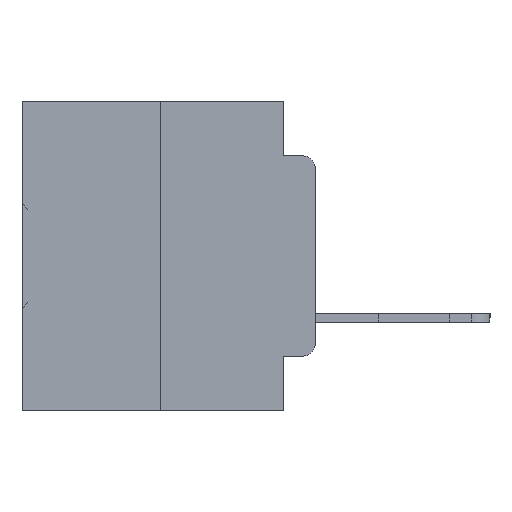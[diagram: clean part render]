
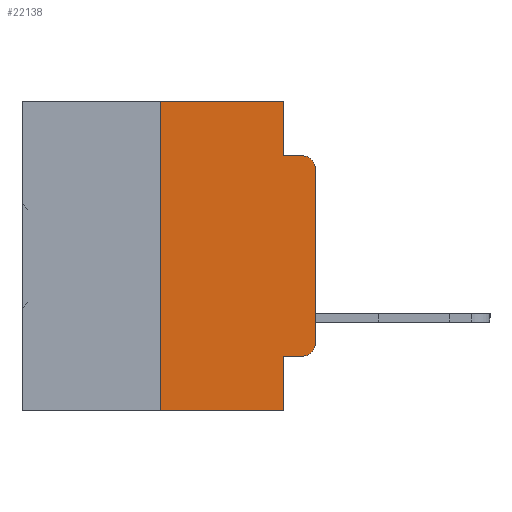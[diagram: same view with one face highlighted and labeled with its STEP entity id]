
A CAD part, left-side view. The second image highlights one B-rep face of the part: STEP entity #22138.
In plain terms, the highlighted planar face has unit normal (-1, 0, 0).
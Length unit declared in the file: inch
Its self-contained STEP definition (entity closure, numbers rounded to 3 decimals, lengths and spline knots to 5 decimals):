
#580 = EDGE_CURVE ( 'NONE', #10509, #17704, #13970, .T. ) ;
#830 = DIRECTION ( 'NONE',  ( -1., 0., 0. ) ) ;
#951 = CARTESIAN_POINT ( 'NONE',  ( 0., 0.02, -0.3915 ) ) ;
#1448 = DIRECTION ( 'NONE',  ( 0., -1., 0. ) ) ;
#2131 = CARTESIAN_POINT ( 'NONE',  ( 0., 0.02, -0.4115 ) ) ;
#2895 = ORIENTED_EDGE ( 'NONE', *, *, #25923, .T. ) ;
#2924 = CARTESIAN_POINT ( 'NONE',  ( 0., 0., -0.1085 ) ) ;
#3681 = DIRECTION ( 'NONE',  ( 0., 0., -1. ) ) ;
#4774 = EDGE_CURVE ( 'NONE', #26540, #25588, #20699, .T. ) ;
#5045 = ORIENTED_EDGE ( 'NONE', *, *, #9909, .F. ) ;
#5196 = AXIS2_PLACEMENT_3D ( 'NONE', #951, #20064, #3681 ) ;
#6168 = VERTEX_POINT ( 'NONE', #33645 ) ;
#6640 = CARTESIAN_POINT ( 'NONE',  ( 0., 0.051, -0.0885 ) ) ;
#6739 = DIRECTION ( 'NONE',  ( 0., 0., 1. ) ) ;
#6847 = LINE ( 'NONE', #20016, #34656 ) ;
#6907 = EDGE_CURVE ( 'NONE', #20873, #34679, #17604, .T. ) ;
#7668 = ORIENTED_EDGE ( 'NONE', *, *, #33949, .F. ) ;
#7806 = LINE ( 'NONE', #27912, #21412 ) ;
#9909 = EDGE_CURVE ( 'NONE', #29156, #6168, #7806, .T. ) ;
#10174 = CARTESIAN_POINT ( 'NONE',  ( 0., 0.051, -0.5 ) ) ;
#10509 = VERTEX_POINT ( 'NONE', #30494 ) ;
#11052 = CIRCLE ( 'NONE', #5196, 0.02 ) ;
#11458 = LINE ( 'NONE', #31200, #24952 ) ;
#12085 = CARTESIAN_POINT ( 'NONE',  ( 0., 0.473, 0. ) ) ;
#12644 = VECTOR ( 'NONE', #6739, 39.37008 ) ;
#13255 = EDGE_CURVE ( 'NONE', #6168, #20873, #11458, .T. ) ;
#13520 = CARTESIAN_POINT ( 'NONE',  ( 0., 0.25, 0. ) ) ;
#13668 = ORIENTED_EDGE ( 'NONE', *, *, #33540, .T. ) ;
#13970 = LINE ( 'NONE', #15401, #29102 ) ;
#14832 = DIRECTION ( 'NONE',  ( 1., 0., 0. ) ) ;
#15401 = CARTESIAN_POINT ( 'NONE',  ( 0., 0.473, -0.5 ) ) ;
#15784 = ORIENTED_EDGE ( 'NONE', *, *, #32378, .F. ) ;
#15901 = VECTOR ( 'NONE', #25900, 39.37008 ) ;
#16081 = ORIENTED_EDGE ( 'NONE', *, *, #17423, .T. ) ;
#16259 = DIRECTION ( 'NONE',  ( 0., 0., 1. ) ) ;
#17233 = CARTESIAN_POINT ( 'NONE',  ( 0., 0.02, -0.1085 ) ) ;
#17407 = VECTOR ( 'NONE', #16259, 39.37008 ) ;
#17423 = EDGE_CURVE ( 'NONE', #25588, #34679, #34330, .T. ) ;
#17454 = DIRECTION ( 'NONE',  ( 0., -1., 0. ) ) ;
#17604 = LINE ( 'NONE', #17841, #15901 ) ;
#17704 = VERTEX_POINT ( 'NONE', #10174 ) ;
#17841 = CARTESIAN_POINT ( 'NONE',  ( 0., 0.051, -0.0885 ) ) ;
#18745 = ORIENTED_EDGE ( 'NONE', *, *, #13255, .F. ) ;
#19548 = ORIENTED_EDGE ( 'NONE', *, *, #6907, .F. ) ;
#19931 = DIRECTION ( 'NONE',  ( 0., 0., -1. ) ) ;
#19958 = EDGE_LOOP ( 'NONE', ( #34484, #16081, #19548, #18745, #5045, #7668, #29201, #15784, #2895, #13668 ) ) ;
#20016 = CARTESIAN_POINT ( 'NONE',  ( 0., 0.051, 0. ) ) ;
#20064 = DIRECTION ( 'NONE',  ( -1., 0., 0. ) ) ;
#20319 = CARTESIAN_POINT ( 'NONE',  ( 0., 0., 0. ) ) ;
#20699 = LINE ( 'NONE', #20319, #12644 ) ;
#20700 = CARTESIAN_POINT ( 'NONE',  ( 0., 0.051, -0.4115 ) ) ;
#20873 = VERTEX_POINT ( 'NONE', #6640 ) ;
#21412 = VECTOR ( 'NONE', #33291, 39.37008 ) ;
#22138 = ADVANCED_FACE ( 'NONE', ( #26741 ), #30798, .F. ) ;
#22362 = VECTOR ( 'NONE', #17454, 39.37008 ) ;
#22830 = DIRECTION ( 'NONE',  ( 0., 0., -1. ) ) ;
#24526 = LINE ( 'NONE', #13520, #17407 ) ;
#24952 = VECTOR ( 'NONE', #33846, 39.37008 ) ;
#25272 = CARTESIAN_POINT ( 'NONE',  ( 0., 0.02, -0.0885 ) ) ;
#25588 = VERTEX_POINT ( 'NONE', #2924 ) ;
#25603 = AXIS2_PLACEMENT_3D ( 'NONE', #12085, #14832, #33545 ) ;
#25900 = DIRECTION ( 'NONE',  ( 0., -1., 0. ) ) ;
#25923 = EDGE_CURVE ( 'NONE', #32507, #30167, #29452, .T. ) ;
#26540 = VERTEX_POINT ( 'NONE', #33523 ) ;
#26741 = FACE_OUTER_BOUND ( 'NONE', #19958, .T. ) ;
#27790 = CARTESIAN_POINT ( 'NONE',  ( 0., 0.25, 0. ) ) ;
#27912 = CARTESIAN_POINT ( 'NONE',  ( 0., 0.473, 0. ) ) ;
#28824 = AXIS2_PLACEMENT_3D ( 'NONE', #17233, #830, #19931 ) ;
#29102 = VECTOR ( 'NONE', #1448, 39.37008 ) ;
#29156 = VERTEX_POINT ( 'NONE', #27790 ) ;
#29201 = ORIENTED_EDGE ( 'NONE', *, *, #580, .T. ) ;
#29452 = LINE ( 'NONE', #33455, #22362 ) ;
#30167 = VERTEX_POINT ( 'NONE', #2131 ) ;
#30494 = CARTESIAN_POINT ( 'NONE',  ( 0., 0.25, -0.5 ) ) ;
#30798 = PLANE ( 'NONE',  #25603 ) ;
#31200 = CARTESIAN_POINT ( 'NONE',  ( 0., 0.051, 0. ) ) ;
#32378 = EDGE_CURVE ( 'NONE', #32507, #17704, #6847, .T. ) ;
#32507 = VERTEX_POINT ( 'NONE', #20700 ) ;
#33291 = DIRECTION ( 'NONE',  ( 0., -1., 0. ) ) ;
#33455 = CARTESIAN_POINT ( 'NONE',  ( 0., 0.051, -0.4115 ) ) ;
#33523 = CARTESIAN_POINT ( 'NONE',  ( 0., 0., -0.3915 ) ) ;
#33540 = EDGE_CURVE ( 'NONE', #30167, #26540, #11052, .T. ) ;
#33545 = DIRECTION ( 'NONE',  ( 0., 0., -1. ) ) ;
#33645 = CARTESIAN_POINT ( 'NONE',  ( 0., 0.051, 0. ) ) ;
#33846 = DIRECTION ( 'NONE',  ( 0., 0., -1. ) ) ;
#33949 = EDGE_CURVE ( 'NONE', #10509, #29156, #24526, .T. ) ;
#34330 = CIRCLE ( 'NONE', #28824, 0.02 ) ;
#34484 = ORIENTED_EDGE ( 'NONE', *, *, #4774, .T. ) ;
#34656 = VECTOR ( 'NONE', #22830, 39.37008 ) ;
#34679 = VERTEX_POINT ( 'NONE', #25272 ) ;
